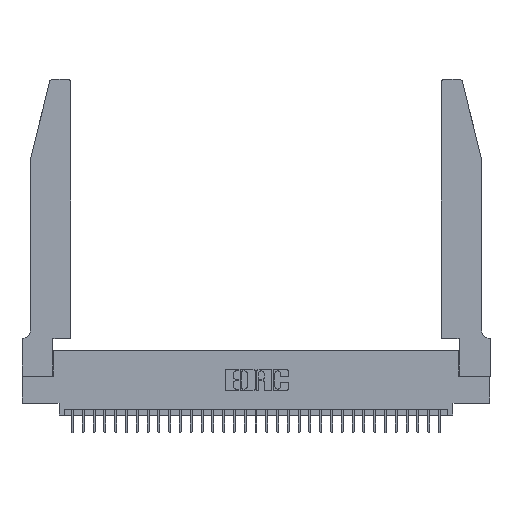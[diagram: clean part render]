
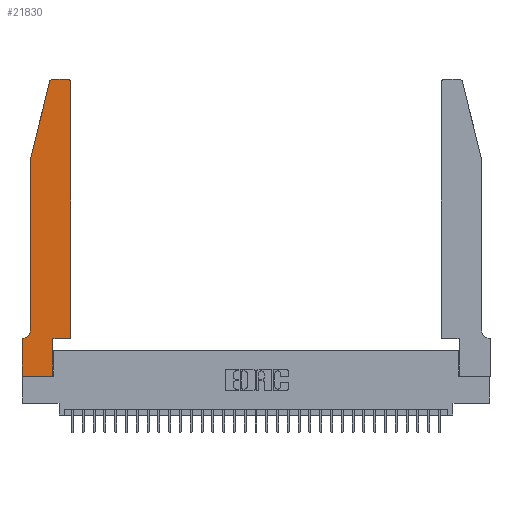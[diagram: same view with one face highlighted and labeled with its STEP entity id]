
A CAD part, top view. The second image highlights one B-rep face of the part: STEP entity #21830.
In plain terms, the highlighted planar face has unit normal (0, 0, 1).
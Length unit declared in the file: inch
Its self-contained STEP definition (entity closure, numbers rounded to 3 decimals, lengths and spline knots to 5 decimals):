
#1029 = CARTESIAN_POINT ( 'NONE',  ( 0.2865, 0.35, 0.37 ) ) ;
#1523 = EDGE_CURVE ( 'NONE', #13174, #15230, #2694, .T. ) ;
#2470 = VECTOR ( 'NONE', #4915, 39.37008 ) ;
#2694 = LINE ( 'NONE', #7387, #20893 ) ;
#3316 = LINE ( 'NONE', #17782, #2470 ) ;
#3568 = CARTESIAN_POINT ( 'NONE',  ( 0.0755, 2., 0.37 ) ) ;
#3584 = ORIENTED_EDGE ( 'NONE', *, *, #1523, .T. ) ;
#3834 = CARTESIAN_POINT ( 'NONE',  ( 0.25487, 2.72718, 0.37 ) ) ;
#4086 = VERTEX_POINT ( 'NONE', #20370 ) ;
#4115 = VERTEX_POINT ( 'NONE', #4953 ) ;
#4501 = DIRECTION ( 'NONE',  ( 1., 0., 0. ) ) ;
#4647 = DIRECTION ( 'NONE',  ( -1., 0., 0. ) ) ;
#4903 = CARTESIAN_POINT ( 'NONE',  ( 0., 0.35, 0.37 ) ) ;
#4915 = DIRECTION ( 'NONE',  ( 0., -1., 0. ) ) ;
#4953 = CARTESIAN_POINT ( 'NONE',  ( 0.2865, 0., 0.37 ) ) ;
#5195 = VERTEX_POINT ( 'NONE', #6471 ) ;
#5476 = LINE ( 'NONE', #25961, #25101 ) ;
#6445 = ORIENTED_EDGE ( 'NONE', *, *, #25218, .T. ) ;
#6471 = CARTESIAN_POINT ( 'NONE',  ( 0.4505, 2.72, 0.37 ) ) ;
#6616 = CARTESIAN_POINT ( 'NONE',  ( 0., 0., 0.37 ) ) ;
#6661 = ORIENTED_EDGE ( 'NONE', *, *, #7015, .T. ) ;
#6949 = CIRCLE ( 'NONE', #21918, 0.03 ) ;
#7015 = EDGE_CURVE ( 'NONE', #5195, #25973, #6949, .T. ) ;
#7387 = CARTESIAN_POINT ( 'NONE',  ( 0.0755, 2., 0.37 ) ) ;
#7844 = ORIENTED_EDGE ( 'NONE', *, *, #14959, .T. ) ;
#9167 = EDGE_CURVE ( 'NONE', #26594, #4115, #11771, .T. ) ;
#9325 = DIRECTION ( 'NONE',  ( 0., 0., 1. ) ) ;
#10115 = DIRECTION ( 'NONE',  ( 1., 0., 0. ) ) ;
#10358 = ORIENTED_EDGE ( 'NONE', *, *, #14014, .T. ) ;
#10381 = CARTESIAN_POINT ( 'NONE',  ( 0.2865, 0.35, 0.37 ) ) ;
#10387 = CARTESIAN_POINT ( 'NONE',  ( 0.4505, 0.35, 0.37 ) ) ;
#11072 = CARTESIAN_POINT ( 'NONE',  ( 0.0055, 0.42, 0.37 ) ) ;
#11080 = VERTEX_POINT ( 'NONE', #10387 ) ;
#11688 = AXIS2_PLACEMENT_3D ( 'NONE', #4903, #25392, #10115 ) ;
#11771 = LINE ( 'NONE', #6616, #31324 ) ;
#12133 = VECTOR ( 'NONE', #4501, 39.37008 ) ;
#12698 = LINE ( 'NONE', #30553, #33035 ) ;
#13116 = DIRECTION ( 'NONE',  ( 0., 0., 1. ) ) ;
#13174 = VERTEX_POINT ( 'NONE', #3568 ) ;
#13667 = DIRECTION ( 'NONE',  ( -1., 0., 0. ) ) ;
#14014 = EDGE_CURVE ( 'NONE', #20036, #26594, #3316, .T. ) ;
#14453 = VERTEX_POINT ( 'NONE', #3834 ) ;
#14959 = EDGE_CURVE ( 'NONE', #15230, #29767, #32535, .T. ) ;
#15230 = VERTEX_POINT ( 'NONE', #29910 ) ;
#15307 = VECTOR ( 'NONE', #30793, 39.37008 ) ;
#15744 = EDGE_CURVE ( 'NONE', #4115, #28449, #24494, .T. ) ;
#16481 = ORIENTED_EDGE ( 'NONE', *, *, #9167, .T. ) ;
#16576 = CARTESIAN_POINT ( 'NONE',  ( 0., 0.35, 0.37 ) ) ;
#16988 = ORIENTED_EDGE ( 'NONE', *, *, #17225, .T. ) ;
#17225 = EDGE_CURVE ( 'NONE', #25973, #4086, #33163, .T. ) ;
#17782 = CARTESIAN_POINT ( 'NONE',  ( 0., 0., 0.37 ) ) ;
#18708 = CARTESIAN_POINT ( 'NONE',  ( 0.4205, 2.75, 0.37 ) ) ;
#18902 = ORIENTED_EDGE ( 'NONE', *, *, #15744, .T. ) ;
#18904 = CARTESIAN_POINT ( 'NONE',  ( 0., 0., 0.37 ) ) ;
#19005 = LINE ( 'NONE', #30052, #12133 ) ;
#20036 = VERTEX_POINT ( 'NONE', #16576 ) ;
#20329 = PLANE ( 'NONE',  #11688 ) ;
#20358 = AXIS2_PLACEMENT_3D ( 'NONE', #11072, #28910, #13667 ) ;
#20359 = EDGE_CURVE ( 'NONE', #29767, #20036, #12698, .T. ) ;
#20370 = CARTESIAN_POINT ( 'NONE',  ( 0.284, 2.75, 0.37 ) ) ;
#20893 = VECTOR ( 'NONE', #22311, 39.37008 ) ;
#21412 = AXIS2_PLACEMENT_3D ( 'NONE', #28355, #13116, #30947 ) ;
#21830 = ADVANCED_FACE ( 'NONE', ( #28121 ), #20329, .T. ) ;
#21918 = AXIS2_PLACEMENT_3D ( 'NONE', #24618, #9325, #27151 ) ;
#21987 = DIRECTION ( 'NONE',  ( 1., 0., 0. ) ) ;
#22311 = DIRECTION ( 'NONE',  ( 0., -1., 0. ) ) ;
#22358 = EDGE_CURVE ( 'NONE', #28449, #11080, #19005, .T. ) ;
#22651 = CARTESIAN_POINT ( 'NONE',  ( 0.2605, 2.75, 0.37 ) ) ;
#24494 = LINE ( 'NONE', #10381, #15307 ) ;
#24570 = EDGE_LOOP ( 'NONE', ( #16988, #6445, #26750, #3584, #7844, #27029, #10358, #16481, #18902, #30758, #30630, #6661 ) ) ;
#24618 = CARTESIAN_POINT ( 'NONE',  ( 0.4205, 2.72, 0.37 ) ) ;
#25101 = VECTOR ( 'NONE', #28517, 39.37008 ) ;
#25218 = EDGE_CURVE ( 'NONE', #4086, #14453, #28282, .T. ) ;
#25392 = DIRECTION ( 'NONE',  ( 0., 0., 1. ) ) ;
#25961 = CARTESIAN_POINT ( 'NONE',  ( 0.0755, 2., 0.37 ) ) ;
#25973 = VERTEX_POINT ( 'NONE', #18708 ) ;
#26377 = LINE ( 'NONE', #32315, #32371 ) ;
#26387 = VECTOR ( 'NONE', #4647, 39.37008 ) ;
#26435 = EDGE_CURVE ( 'NONE', #14453, #13174, #5476, .T. ) ;
#26594 = VERTEX_POINT ( 'NONE', #18904 ) ;
#26750 = ORIENTED_EDGE ( 'NONE', *, *, #26435, .T. ) ;
#26800 = EDGE_CURVE ( 'NONE', #11080, #5195, #26377, .T. ) ;
#27029 = ORIENTED_EDGE ( 'NONE', *, *, #20359, .T. ) ;
#27151 = DIRECTION ( 'NONE',  ( 1., 0., 0. ) ) ;
#27954 = DIRECTION ( 'NONE',  ( -1., 0., 0. ) ) ;
#28121 = FACE_OUTER_BOUND ( 'NONE', #24570, .T. ) ;
#28282 = CIRCLE ( 'NONE', #21412, 0.03 ) ;
#28355 = CARTESIAN_POINT ( 'NONE',  ( 0.284, 2.72, 0.37 ) ) ;
#28449 = VERTEX_POINT ( 'NONE', #1029 ) ;
#28517 = DIRECTION ( 'NONE',  ( -0.239, -0.971, 0. ) ) ;
#28910 = DIRECTION ( 'NONE',  ( 0., 0., -1. ) ) ;
#29767 = VERTEX_POINT ( 'NONE', #32064 ) ;
#29910 = CARTESIAN_POINT ( 'NONE',  ( 0.0755, 0.42, 0.37 ) ) ;
#30052 = CARTESIAN_POINT ( 'NONE',  ( 0.4505, 0.35, 0.37 ) ) ;
#30553 = CARTESIAN_POINT ( 'NONE',  ( 0.0755, 0.35, 0.37 ) ) ;
#30630 = ORIENTED_EDGE ( 'NONE', *, *, #26800, .T. ) ;
#30758 = ORIENTED_EDGE ( 'NONE', *, *, #22358, .T. ) ;
#30793 = DIRECTION ( 'NONE',  ( 0., 1., 0. ) ) ;
#30947 = DIRECTION ( 'NONE',  ( 1., 0., 0. ) ) ;
#31324 = VECTOR ( 'NONE', #21987, 39.37008 ) ;
#32064 = CARTESIAN_POINT ( 'NONE',  ( 0.0055, 0.35, 0.37 ) ) ;
#32315 = CARTESIAN_POINT ( 'NONE',  ( 0.4505, 0.35, 0.37 ) ) ;
#32371 = VECTOR ( 'NONE', #32425, 39.37008 ) ;
#32425 = DIRECTION ( 'NONE',  ( 0., 1., 0. ) ) ;
#32535 = CIRCLE ( 'NONE', #20358, 0.07 ) ;
#33035 = VECTOR ( 'NONE', #27954, 39.37008 ) ;
#33163 = LINE ( 'NONE', #22651, #26387 ) ;
